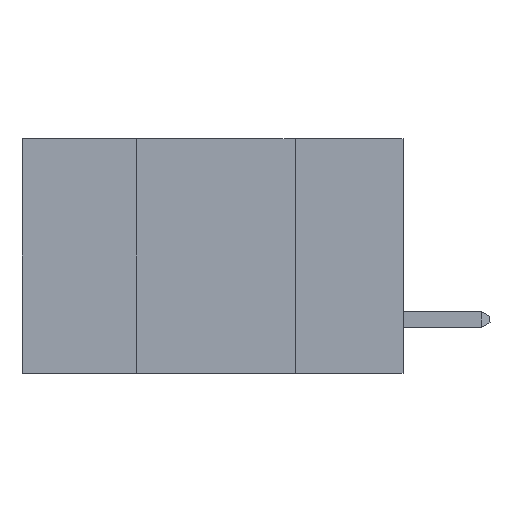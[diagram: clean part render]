
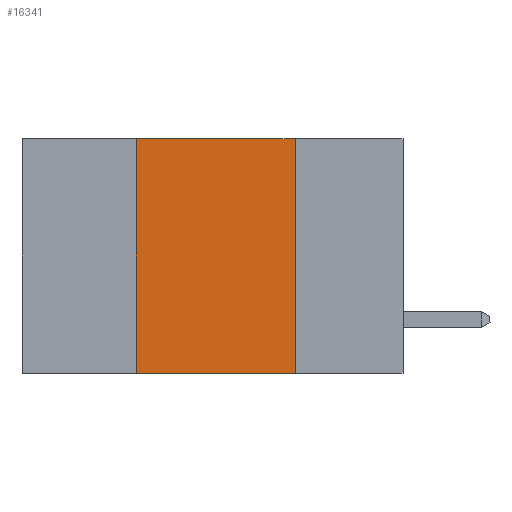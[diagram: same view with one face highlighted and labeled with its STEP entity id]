
A CAD part, left-side view. The second image highlights one B-rep face of the part: STEP entity #16341.
In plain terms, the highlighted planar face has unit normal (-1, 0, 0).
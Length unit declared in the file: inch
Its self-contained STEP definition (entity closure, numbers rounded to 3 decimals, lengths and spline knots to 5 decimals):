
#1742 = DIRECTION ( 'NONE',  ( 0., -1., 0. ) ) ;
#2191 = VERTEX_POINT ( 'NONE', #16511 ) ;
#2829 = EDGE_CURVE ( 'NONE', #10729, #9931, #15724, .T. ) ;
#3440 = EDGE_LOOP ( 'NONE', ( #7101, #15405, #7317, #18788 ) ) ;
#3857 = LINE ( 'NONE', #9185, #18165 ) ;
#4244 = DIRECTION ( 'NONE',  ( 1., 0., 0. ) ) ;
#4516 = EDGE_CURVE ( 'NONE', #18705, #9931, #6002, .T. ) ;
#4969 = DIRECTION ( 'NONE',  ( 0., -1., 0. ) ) ;
#5151 = CARTESIAN_POINT ( 'NONE',  ( 0., 0.6, -0.37 ) ) ;
#5329 = CARTESIAN_POINT ( 'NONE',  ( 0., 0.42, -0.37 ) ) ;
#5529 = EDGE_CURVE ( 'NONE', #10729, #2191, #7641, .T. ) ;
#6002 = LINE ( 'NONE', #9930, #13729 ) ;
#7101 = ORIENTED_EDGE ( 'NONE', *, *, #4516, .F. ) ;
#7317 = ORIENTED_EDGE ( 'NONE', *, *, #5529, .F. ) ;
#7641 = LINE ( 'NONE', #10075, #15700 ) ;
#7779 = AXIS2_PLACEMENT_3D ( 'NONE', #8623, #4244, #14436 ) ;
#8623 = CARTESIAN_POINT ( 'NONE',  ( 0., 0.6, 0. ) ) ;
#9185 = CARTESIAN_POINT ( 'NONE',  ( 0., 0.6, 0. ) ) ;
#9930 = CARTESIAN_POINT ( 'NONE',  ( 0., 0.17, 0. ) ) ;
#9931 = VERTEX_POINT ( 'NONE', #12185 ) ;
#9953 = DIRECTION ( 'NONE',  ( 0., 0., -1. ) ) ;
#10037 = DIRECTION ( 'NONE',  ( 0., 0., 1. ) ) ;
#10075 = CARTESIAN_POINT ( 'NONE',  ( 0., 0.42, 0. ) ) ;
#10729 = VERTEX_POINT ( 'NONE', #5329 ) ;
#12006 = VECTOR ( 'NONE', #4969, 39.37008 ) ;
#12185 = CARTESIAN_POINT ( 'NONE',  ( 0., 0.17, -0.37 ) ) ;
#13031 = PLANE ( 'NONE',  #7779 ) ;
#13729 = VECTOR ( 'NONE', #9953, 39.37008 ) ;
#14194 = CARTESIAN_POINT ( 'NONE',  ( 0., 0.17, 0. ) ) ;
#14436 = DIRECTION ( 'NONE',  ( 0., 0., -1. ) ) ;
#15219 = FACE_OUTER_BOUND ( 'NONE', #3440, .T. ) ;
#15405 = ORIENTED_EDGE ( 'NONE', *, *, #16575, .F. ) ;
#15700 = VECTOR ( 'NONE', #10037, 39.37008 ) ;
#15724 = LINE ( 'NONE', #5151, #12006 ) ;
#16341 = ADVANCED_FACE ( 'NONE', ( #15219 ), #13031, .F. ) ;
#16511 = CARTESIAN_POINT ( 'NONE',  ( 0., 0.42, 0. ) ) ;
#16575 = EDGE_CURVE ( 'NONE', #2191, #18705, #3857, .T. ) ;
#18165 = VECTOR ( 'NONE', #1742, 39.37008 ) ;
#18705 = VERTEX_POINT ( 'NONE', #14194 ) ;
#18788 = ORIENTED_EDGE ( 'NONE', *, *, #2829, .T. ) ;
